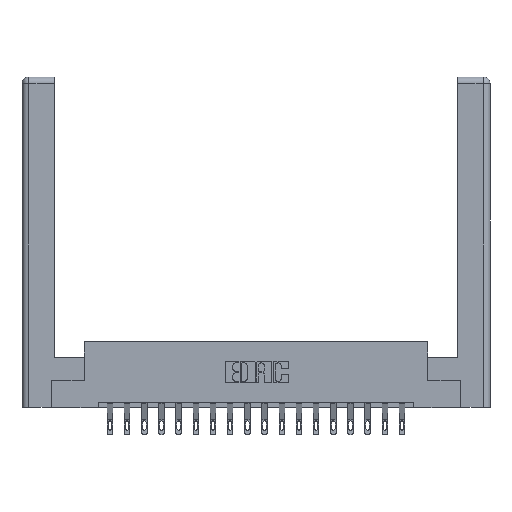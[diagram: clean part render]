
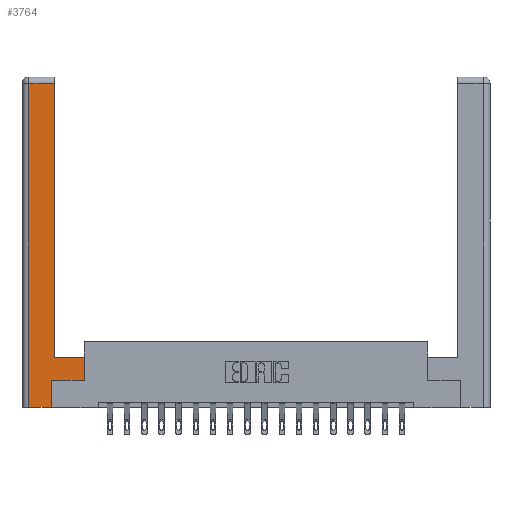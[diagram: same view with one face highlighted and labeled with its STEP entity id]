
A CAD part, top view. The second image highlights one B-rep face of the part: STEP entity #3764.
In plain terms, the highlighted planar face has unit normal (0, 0, 1).
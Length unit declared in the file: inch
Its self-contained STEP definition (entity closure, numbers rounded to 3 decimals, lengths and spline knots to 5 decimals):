
#146 = ORIENTED_EDGE ( 'NONE', *, *, #7924, .T. ) ;
#402 = VECTOR ( 'NONE', #19547, 39.37008 ) ;
#2114 = ORIENTED_EDGE ( 'NONE', *, *, #5820, .T. ) ;
#2247 = CARTESIAN_POINT ( 'NONE',  ( 0.265, 0.245, 0. ) ) ;
#2295 = DIRECTION ( 'NONE',  ( 1., 0., 0. ) ) ;
#2464 = LINE ( 'NONE', #12231, #19410 ) ;
#2597 = ORIENTED_EDGE ( 'NONE', *, *, #10205, .T. ) ;
#2708 = CARTESIAN_POINT ( 'NONE',  ( 0.0615, 0., 0. ) ) ;
#3269 = CARTESIAN_POINT ( 'NONE',  ( 0.565, 0.245, 0. ) ) ;
#3300 = VECTOR ( 'NONE', #12143, 39.37008 ) ;
#3361 = VERTEX_POINT ( 'NONE', #14166 ) ;
#3630 = ORIENTED_EDGE ( 'NONE', *, *, #8666, .T. ) ;
#3764 = ADVANCED_FACE ( 'NONE', ( #12392 ), #5352, .F. ) ;
#5352 = PLANE ( 'NONE',  #19020 ) ;
#5820 = EDGE_CURVE ( 'NONE', #18662, #10447, #14646, .T. ) ;
#6206 = ORIENTED_EDGE ( 'NONE', *, *, #12526, .T. ) ;
#6791 = CARTESIAN_POINT ( 'NONE',  ( 0.565, 0.245, 0. ) ) ;
#7028 = DIRECTION ( 'NONE',  ( 0., 0., -1. ) ) ;
#7260 = CARTESIAN_POINT ( 'NONE',  ( 0.265, 0., 0. ) ) ;
#7312 = LINE ( 'NONE', #7260, #19877 ) ;
#7924 = EDGE_CURVE ( 'NONE', #13211, #12506, #12427, .T. ) ;
#8460 = DIRECTION ( 'NONE',  ( 0., 1., 0. ) ) ;
#8666 = EDGE_CURVE ( 'NONE', #10447, #13211, #2464, .T. ) ;
#8825 = DIRECTION ( 'NONE',  ( 1., 0., 0. ) ) ;
#8986 = DIRECTION ( 'NONE',  ( 0., -1., 0. ) ) ;
#9533 = EDGE_CURVE ( 'NONE', #10744, #3361, #17943, .T. ) ;
#9979 = CARTESIAN_POINT ( 'NONE',  ( 0.0615, 2.94, 0. ) ) ;
#10135 = DIRECTION ( 'NONE',  ( -1., 0., 0. ) ) ;
#10205 = EDGE_CURVE ( 'NONE', #3361, #18662, #15946, .T. ) ;
#10447 = VERTEX_POINT ( 'NONE', #13575 ) ;
#10472 = CARTESIAN_POINT ( 'NONE',  ( 0.295, 2.94, 0. ) ) ;
#10744 = VERTEX_POINT ( 'NONE', #13355 ) ;
#10821 = DIRECTION ( 'NONE',  ( 0., 1., 0. ) ) ;
#10925 = VECTOR ( 'NONE', #8460, 39.37008 ) ;
#11701 = EDGE_CURVE ( 'NONE', #12687, #10744, #7312, .T. ) ;
#12143 = DIRECTION ( 'NONE',  ( 0., 1., 0. ) ) ;
#12231 = CARTESIAN_POINT ( 'NONE',  ( 0.295, 0.45, 0. ) ) ;
#12351 = VECTOR ( 'NONE', #8986, 39.37008 ) ;
#12392 = FACE_OUTER_BOUND ( 'NONE', #13772, .T. ) ;
#12427 = LINE ( 'NONE', #18181, #13156 ) ;
#12506 = VERTEX_POINT ( 'NONE', #10472 ) ;
#12526 = EDGE_CURVE ( 'NONE', #16466, #12687, #16477, .T. ) ;
#12559 = VECTOR ( 'NONE', #2295, 39.37008 ) ;
#12687 = VERTEX_POINT ( 'NONE', #2708 ) ;
#13156 = VECTOR ( 'NONE', #10821, 39.37008 ) ;
#13211 = VERTEX_POINT ( 'NONE', #16763 ) ;
#13355 = CARTESIAN_POINT ( 'NONE',  ( 0.265, 0., 0. ) ) ;
#13575 = CARTESIAN_POINT ( 'NONE',  ( 0.565, 0.45, 0. ) ) ;
#13772 = EDGE_LOOP ( 'NONE', ( #146, #18151, #6206, #15430, #15836, #2597, #2114, #3630 ) ) ;
#14166 = CARTESIAN_POINT ( 'NONE',  ( 0.265, 0.245, 0. ) ) ;
#14646 = LINE ( 'NONE', #18379, #3300 ) ;
#14835 = EDGE_CURVE ( 'NONE', #12506, #16466, #17838, .T. ) ;
#15235 = CARTESIAN_POINT ( 'NONE',  ( 0.0615, 0., 0. ) ) ;
#15430 = ORIENTED_EDGE ( 'NONE', *, *, #11701, .T. ) ;
#15836 = ORIENTED_EDGE ( 'NONE', *, *, #9533, .T. ) ;
#15946 = LINE ( 'NONE', #6791, #12559 ) ;
#16129 = CARTESIAN_POINT ( 'NONE',  ( 0., 0., 0. ) ) ;
#16466 = VERTEX_POINT ( 'NONE', #18502 ) ;
#16477 = LINE ( 'NONE', #15235, #12351 ) ;
#16763 = CARTESIAN_POINT ( 'NONE',  ( 0.295, 0.45, 0. ) ) ;
#16845 = DIRECTION ( 'NONE',  ( -1., 0., 0. ) ) ;
#17838 = LINE ( 'NONE', #9979, #402 ) ;
#17943 = LINE ( 'NONE', #2247, #10925 ) ;
#18151 = ORIENTED_EDGE ( 'NONE', *, *, #14835, .T. ) ;
#18181 = CARTESIAN_POINT ( 'NONE',  ( 0.295, 3., 0. ) ) ;
#18379 = CARTESIAN_POINT ( 'NONE',  ( 0.565, 0.45, 0. ) ) ;
#18502 = CARTESIAN_POINT ( 'NONE',  ( 0.0615, 2.94, 0. ) ) ;
#18662 = VERTEX_POINT ( 'NONE', #3269 ) ;
#19020 = AXIS2_PLACEMENT_3D ( 'NONE', #16129, #7028, #10135 ) ;
#19410 = VECTOR ( 'NONE', #16845, 39.37008 ) ;
#19547 = DIRECTION ( 'NONE',  ( -1., 0., 0. ) ) ;
#19877 = VECTOR ( 'NONE', #8825, 39.37008 ) ;
